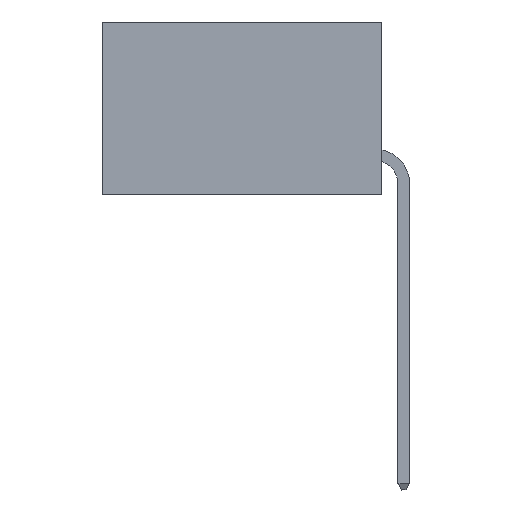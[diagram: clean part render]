
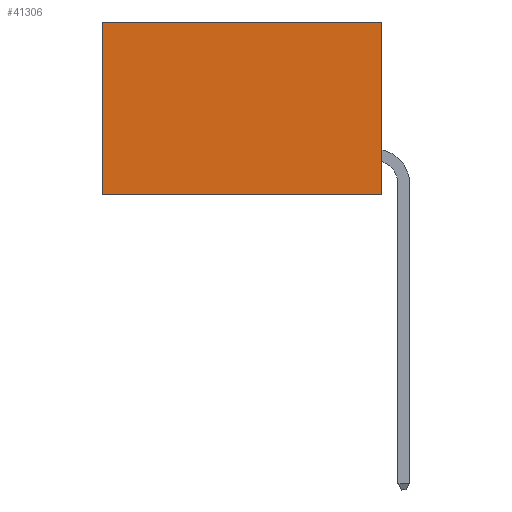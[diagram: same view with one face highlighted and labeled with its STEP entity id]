
A CAD part, left-side view. The second image highlights one B-rep face of the part: STEP entity #41306.
In plain terms, the highlighted planar face has unit normal (-1, 0, 0).
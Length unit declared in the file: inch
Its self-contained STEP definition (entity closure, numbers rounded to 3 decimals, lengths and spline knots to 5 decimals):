
#371 = VECTOR ( 'NONE', #16232, 39.37008 ) ;
#1244 = VERTEX_POINT ( 'NONE', #10894 ) ;
#1439 = VERTEX_POINT ( 'NONE', #15968 ) ;
#1574 = DIRECTION ( 'NONE',  ( 0., 0., -1. ) ) ;
#2428 = CARTESIAN_POINT ( 'NONE',  ( 0.2875, 0., 0. ) ) ;
#5489 = ORIENTED_EDGE ( 'NONE', *, *, #28972, .F. ) ;
#5829 = CARTESIAN_POINT ( 'NONE',  ( 0.2875, 0.6, -0.37 ) ) ;
#8432 = DIRECTION ( 'NONE',  ( 0., 1., 0. ) ) ;
#8637 = ORIENTED_EDGE ( 'NONE', *, *, #31597, .T. ) ;
#8936 = LINE ( 'NONE', #18876, #28460 ) ;
#10510 = VECTOR ( 'NONE', #8432, 39.37008 ) ;
#10894 = CARTESIAN_POINT ( 'NONE',  ( 0.2875, 0.6, 0. ) ) ;
#13818 = AXIS2_PLACEMENT_3D ( 'NONE', #36357, #35909, #1574 ) ;
#15208 = ORIENTED_EDGE ( 'NONE', *, *, #33823, .F. ) ;
#15968 = CARTESIAN_POINT ( 'NONE',  ( 0.2875, 0., -0.37 ) ) ;
#16232 = DIRECTION ( 'NONE',  ( 0., 1., 0. ) ) ;
#18876 = CARTESIAN_POINT ( 'NONE',  ( 0.2875, 0., 0. ) ) ;
#19210 = VERTEX_POINT ( 'NONE', #2428 ) ;
#22278 = EDGE_LOOP ( 'NONE', ( #28130, #5489, #15208, #8637 ) ) ;
#22432 = LINE ( 'NONE', #25693, #10510 ) ;
#23051 = CARTESIAN_POINT ( 'NONE',  ( 0.2875, 0., 0. ) ) ;
#25158 = VERTEX_POINT ( 'NONE', #5829 ) ;
#25693 = CARTESIAN_POINT ( 'NONE',  ( 0.2875, 0., -0.37 ) ) ;
#26007 = DIRECTION ( 'NONE',  ( 0., 0., -1. ) ) ;
#26345 = VECTOR ( 'NONE', #42758, 39.37008 ) ;
#27275 = EDGE_CURVE ( 'NONE', #1244, #25158, #28510, .T. ) ;
#28130 = ORIENTED_EDGE ( 'NONE', *, *, #27275, .T. ) ;
#28460 = VECTOR ( 'NONE', #26007, 39.37008 ) ;
#28510 = LINE ( 'NONE', #39592, #26345 ) ;
#28972 = EDGE_CURVE ( 'NONE', #1439, #25158, #22432, .T. ) ;
#31597 = EDGE_CURVE ( 'NONE', #19210, #1244, #41123, .T. ) ;
#33823 = EDGE_CURVE ( 'NONE', #19210, #1439, #8936, .T. ) ;
#35909 = DIRECTION ( 'NONE',  ( 1., 0., 0. ) ) ;
#36357 = CARTESIAN_POINT ( 'NONE',  ( 0.2875, 0., 0. ) ) ;
#39592 = CARTESIAN_POINT ( 'NONE',  ( 0.2875, 0.6, 0. ) ) ;
#41123 = LINE ( 'NONE', #23051, #371 ) ;
#41306 = ADVANCED_FACE ( 'NONE', ( #41980 ), #43000, .F. ) ;
#41980 = FACE_OUTER_BOUND ( 'NONE', #22278, .T. ) ;
#42758 = DIRECTION ( 'NONE',  ( 0., 0., -1. ) ) ;
#43000 = PLANE ( 'NONE',  #13818 ) ;
